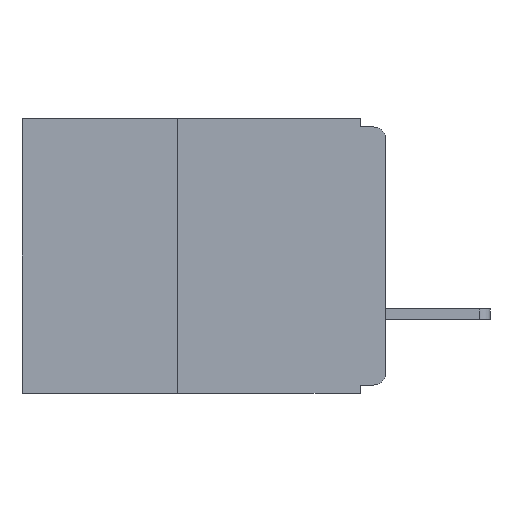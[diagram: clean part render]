
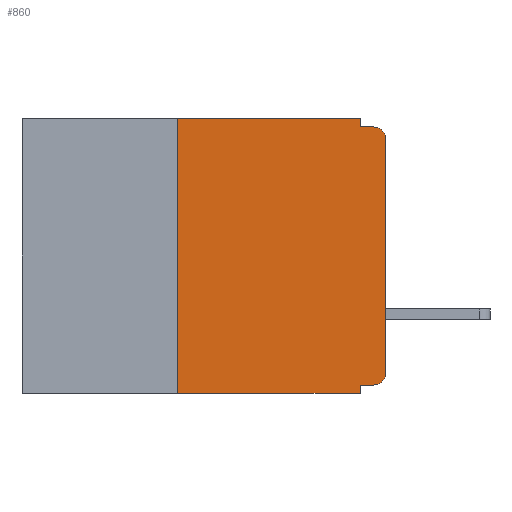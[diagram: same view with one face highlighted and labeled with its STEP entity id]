
A CAD part, left-side view. The second image highlights one B-rep face of the part: STEP entity #860.
In plain terms, the highlighted planar face has unit normal (-1, 0, 0).
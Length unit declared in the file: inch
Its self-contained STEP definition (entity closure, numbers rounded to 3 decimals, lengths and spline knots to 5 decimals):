
#85 = CARTESIAN_POINT ( 'NONE',  ( 0., 0., -0.025 ) ) ;
#122 = VERTEX_POINT ( 'NONE', #8388 ) ;
#127 = EDGE_LOOP ( 'NONE', ( #2717, #2884, #3078, #3093, #3154, #5485, #8319, #8338, #8510, #9031 ) ) ;
#367 = VERTEX_POINT ( 'NONE', #10398 ) ;
#551 = LINE ( 'NONE', #12809, #3532 ) ;
#631 = DIRECTION ( 'NONE',  ( 0., 0., -1. ) ) ;
#860 = ADVANCED_FACE ( 'NONE', ( #13203 ), #2040, .F. ) ;
#880 = EDGE_CURVE ( 'NONE', #3869, #5314, #11084, .T. ) ;
#894 = VERTEX_POINT ( 'NONE', #10141 ) ;
#982 = EDGE_CURVE ( 'NONE', #13778, #4781, #12139, .T. ) ;
#1104 = EDGE_CURVE ( 'NONE', #5144, #122, #11234, .T. ) ;
#1167 = DIRECTION ( 'NONE',  ( 0., 1., 0. ) ) ;
#1177 = EDGE_CURVE ( 'NONE', #5314, #4781, #7757, .T. ) ;
#1285 = EDGE_CURVE ( 'NONE', #5144, #3869, #9046, .T. ) ;
#1286 = DIRECTION ( 'NONE',  ( 0., -1., 0. ) ) ;
#1928 = CARTESIAN_POINT ( 'NONE',  ( 0., 0., -0.305 ) ) ;
#2040 = PLANE ( 'NONE',  #7802 ) ;
#2348 = DIRECTION ( 'NONE',  ( -1., 0., 0. ) ) ;
#2717 = ORIENTED_EDGE ( 'NONE', *, *, #880, .T. ) ;
#2720 = CARTESIAN_POINT ( 'NONE',  ( 0., 0.25, -0.33 ) ) ;
#2884 = ORIENTED_EDGE ( 'NONE', *, *, #1177, .T. ) ;
#2886 = EDGE_CURVE ( 'NONE', #894, #13778, #7338, .T. ) ;
#2932 = EDGE_CURVE ( 'NONE', #5770, #367, #6987, .T. ) ;
#2936 = EDGE_CURVE ( 'NONE', #5770, #5309, #551, .T. ) ;
#2998 = EDGE_CURVE ( 'NONE', #122, #5309, #8249, .T. ) ;
#3078 = ORIENTED_EDGE ( 'NONE', *, *, #982, .F. ) ;
#3093 = ORIENTED_EDGE ( 'NONE', *, *, #2886, .F. ) ;
#3154 = ORIENTED_EDGE ( 'NONE', *, *, #8533, .F. ) ;
#3532 = VECTOR ( 'NONE', #12844, 39.37008 ) ;
#3869 = VERTEX_POINT ( 'NONE', #1928 ) ;
#3894 = LINE ( 'NONE', #4214, #11927 ) ;
#4214 = CARTESIAN_POINT ( 'NONE',  ( 0., 0.437, 0. ) ) ;
#4781 = VERTEX_POINT ( 'NONE', #13393 ) ;
#5093 = VECTOR ( 'NONE', #1167, 39.37008 ) ;
#5144 = VERTEX_POINT ( 'NONE', #10360 ) ;
#5248 = DIRECTION ( 'NONE',  ( 0., 0., -1. ) ) ;
#5309 = VERTEX_POINT ( 'NONE', #8593 ) ;
#5314 = VERTEX_POINT ( 'NONE', #85 ) ;
#5484 = CARTESIAN_POINT ( 'NONE',  ( 0., 0.015, -0.025 ) ) ;
#5485 = ORIENTED_EDGE ( 'NONE', *, *, #2932, .F. ) ;
#5572 = VECTOR ( 'NONE', #11173, 39.37008 ) ;
#5770 = VERTEX_POINT ( 'NONE', #2720 ) ;
#6535 = VECTOR ( 'NONE', #1286, 39.37008 ) ;
#6896 = AXIS2_PLACEMENT_3D ( 'NONE', #11149, #2348, #5248 ) ;
#6987 = LINE ( 'NONE', #12942, #9326 ) ;
#7202 = AXIS2_PLACEMENT_3D ( 'NONE', #5484, #12347, #631 ) ;
#7338 = LINE ( 'NONE', #13981, #9957 ) ;
#7663 = DIRECTION ( 'NONE',  ( 0., -1., 0. ) ) ;
#7757 = CIRCLE ( 'NONE', #7202, 0.015 ) ;
#7802 = AXIS2_PLACEMENT_3D ( 'NONE', #10628, #10733, #7883 ) ;
#7883 = DIRECTION ( 'NONE',  ( 0., 0., -1. ) ) ;
#8038 = CARTESIAN_POINT ( 'NONE',  ( 0., 0., 0. ) ) ;
#8249 = LINE ( 'NONE', #10507, #5572 ) ;
#8319 = ORIENTED_EDGE ( 'NONE', *, *, #2936, .T. ) ;
#8337 = CARTESIAN_POINT ( 'NONE',  ( 0., 0., -0.01 ) ) ;
#8338 = ORIENTED_EDGE ( 'NONE', *, *, #2998, .F. ) ;
#8388 = CARTESIAN_POINT ( 'NONE',  ( 0., 0.031, -0.32 ) ) ;
#8510 = ORIENTED_EDGE ( 'NONE', *, *, #1104, .F. ) ;
#8533 = EDGE_CURVE ( 'NONE', #367, #894, #3894, .T. ) ;
#8593 = CARTESIAN_POINT ( 'NONE',  ( 0., 0.031, -0.33 ) ) ;
#9031 = ORIENTED_EDGE ( 'NONE', *, *, #1285, .T. ) ;
#9046 = CIRCLE ( 'NONE', #6896, 0.015 ) ;
#9326 = VECTOR ( 'NONE', #12998, 39.37008 ) ;
#9957 = VECTOR ( 'NONE', #13883, 39.37008 ) ;
#10141 = CARTESIAN_POINT ( 'NONE',  ( 0., 0.031, 0. ) ) ;
#10360 = CARTESIAN_POINT ( 'NONE',  ( 0., 0.015, -0.32 ) ) ;
#10398 = CARTESIAN_POINT ( 'NONE',  ( 0., 0.25, 0. ) ) ;
#10507 = CARTESIAN_POINT ( 'NONE',  ( 0., 0.031, -0.33 ) ) ;
#10628 = CARTESIAN_POINT ( 'NONE',  ( 0., 0.437, 0. ) ) ;
#10733 = DIRECTION ( 'NONE',  ( 1., 0., 0. ) ) ;
#10771 = VECTOR ( 'NONE', #11734, 39.37008 ) ;
#11084 = LINE ( 'NONE', #8038, #10771 ) ;
#11149 = CARTESIAN_POINT ( 'NONE',  ( 0., 0.015, -0.305 ) ) ;
#11173 = DIRECTION ( 'NONE',  ( 0., 0., -1. ) ) ;
#11234 = LINE ( 'NONE', #13330, #5093 ) ;
#11673 = CARTESIAN_POINT ( 'NONE',  ( 0., 0.031, -0.01 ) ) ;
#11734 = DIRECTION ( 'NONE',  ( 0., 0., 1. ) ) ;
#11927 = VECTOR ( 'NONE', #7663, 39.37008 ) ;
#12139 = LINE ( 'NONE', #8337, #6535 ) ;
#12347 = DIRECTION ( 'NONE',  ( -1., 0., 0. ) ) ;
#12809 = CARTESIAN_POINT ( 'NONE',  ( 0., 0.437, -0.33 ) ) ;
#12844 = DIRECTION ( 'NONE',  ( 0., -1., 0. ) ) ;
#12942 = CARTESIAN_POINT ( 'NONE',  ( 0., 0.25, -0.33 ) ) ;
#12998 = DIRECTION ( 'NONE',  ( 0., 0., 1. ) ) ;
#13203 = FACE_OUTER_BOUND ( 'NONE', #127, .T. ) ;
#13330 = CARTESIAN_POINT ( 'NONE',  ( 0., 0., -0.32 ) ) ;
#13393 = CARTESIAN_POINT ( 'NONE',  ( 0., 0.015, -0.01 ) ) ;
#13778 = VERTEX_POINT ( 'NONE', #11673 ) ;
#13883 = DIRECTION ( 'NONE',  ( 0., 0., -1. ) ) ;
#13981 = CARTESIAN_POINT ( 'NONE',  ( 0., 0.031, 0. ) ) ;
